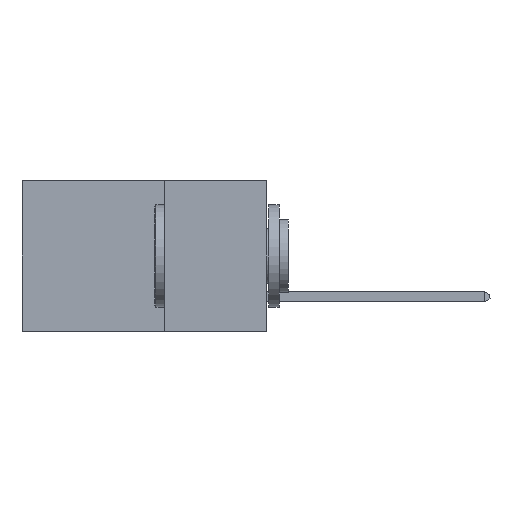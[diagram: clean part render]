
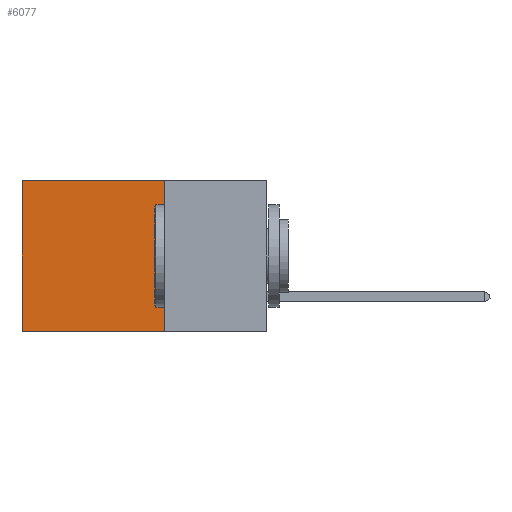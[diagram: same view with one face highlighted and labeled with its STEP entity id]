
A CAD part, left-side view. The second image highlights one B-rep face of the part: STEP entity #6077.
In plain terms, the highlighted planar face has unit normal (-1, 0, 0).
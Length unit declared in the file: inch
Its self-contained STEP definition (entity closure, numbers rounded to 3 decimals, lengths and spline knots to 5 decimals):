
#291 = DIRECTION ( 'NONE',  ( 0., 0., -1. ) ) ;
#548 = LINE ( 'NONE', #6794, #8297 ) ;
#579 = VERTEX_POINT ( 'NONE', #12974 ) ;
#2630 = ORIENTED_EDGE ( 'NONE', *, *, #10350, .F. ) ;
#2779 = LINE ( 'NONE', #15027, #20026 ) ;
#3246 = DIRECTION ( 'NONE',  ( 0., 1., 0. ) ) ;
#5007 = VERTEX_POINT ( 'NONE', #17671 ) ;
#6077 = ADVANCED_FACE ( 'NONE', ( #17144 ), #7347, .F. ) ;
#6245 = CARTESIAN_POINT ( 'NONE',  ( 0.2875, 0.25, -0.37 ) ) ;
#6794 = CARTESIAN_POINT ( 'NONE',  ( 0.2875, 0.6, 0. ) ) ;
#7347 = PLANE ( 'NONE',  #16844 ) ;
#7450 = EDGE_CURVE ( 'NONE', #579, #20877, #548, .T. ) ;
#8068 = EDGE_CURVE ( 'NONE', #11224, #20877, #15024, .T. ) ;
#8297 = VECTOR ( 'NONE', #13542, 39.37008 ) ;
#8662 = EDGE_CURVE ( 'NONE', #5007, #579, #2779, .T. ) ;
#9647 = EDGE_LOOP ( 'NONE', ( #18049, #16658, #2630, #13269 ) ) ;
#10105 = CARTESIAN_POINT ( 'NONE',  ( 0.2875, 0.25, -0.37 ) ) ;
#10350 = EDGE_CURVE ( 'NONE', #5007, #11224, #11145, .T. ) ;
#10723 = DIRECTION ( 'NONE',  ( 1., 0., 0. ) ) ;
#10832 = DIRECTION ( 'NONE',  ( 0., 0., -1. ) ) ;
#11145 = LINE ( 'NONE', #14104, #15589 ) ;
#11224 = VERTEX_POINT ( 'NONE', #6245 ) ;
#12974 = CARTESIAN_POINT ( 'NONE',  ( 0.2875, 0.6, 0. ) ) ;
#13269 = ORIENTED_EDGE ( 'NONE', *, *, #8662, .T. ) ;
#13542 = DIRECTION ( 'NONE',  ( 0., 0., -1. ) ) ;
#14104 = CARTESIAN_POINT ( 'NONE',  ( 0.2875, 0.25, 0. ) ) ;
#15024 = LINE ( 'NONE', #10105, #18311 ) ;
#15027 = CARTESIAN_POINT ( 'NONE',  ( 0.2875, 0.25, 0. ) ) ;
#15589 = VECTOR ( 'NONE', #10832, 39.37008 ) ;
#16658 = ORIENTED_EDGE ( 'NONE', *, *, #8068, .F. ) ;
#16760 = DIRECTION ( 'NONE',  ( 0., 1., 0. ) ) ;
#16844 = AXIS2_PLACEMENT_3D ( 'NONE', #20493, #10723, #291 ) ;
#16976 = CARTESIAN_POINT ( 'NONE',  ( 0.2875, 0.6, -0.37 ) ) ;
#17144 = FACE_OUTER_BOUND ( 'NONE', #9647, .T. ) ;
#17671 = CARTESIAN_POINT ( 'NONE',  ( 0.2875, 0.25, 0. ) ) ;
#18049 = ORIENTED_EDGE ( 'NONE', *, *, #7450, .T. ) ;
#18311 = VECTOR ( 'NONE', #16760, 39.37008 ) ;
#20026 = VECTOR ( 'NONE', #3246, 39.37008 ) ;
#20493 = CARTESIAN_POINT ( 'NONE',  ( 0.2875, 0.25, 0. ) ) ;
#20877 = VERTEX_POINT ( 'NONE', #16976 ) ;
